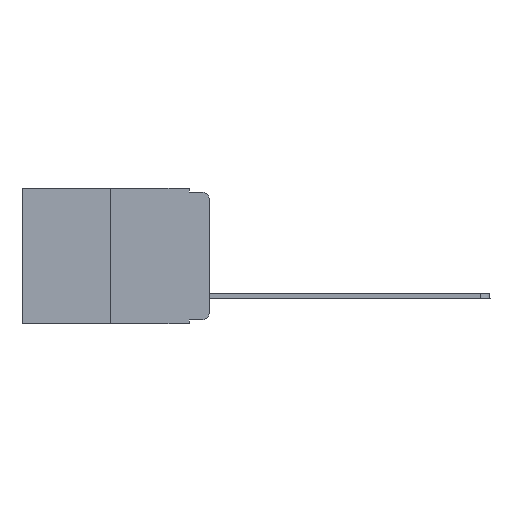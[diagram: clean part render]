
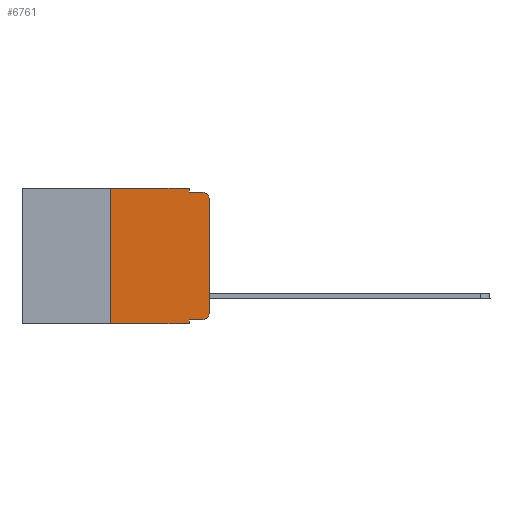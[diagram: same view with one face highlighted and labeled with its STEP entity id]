
A CAD part, left-side view. The second image highlights one B-rep face of the part: STEP entity #6761.
In plain terms, the highlighted planar face has unit normal (-1, 0, 0).
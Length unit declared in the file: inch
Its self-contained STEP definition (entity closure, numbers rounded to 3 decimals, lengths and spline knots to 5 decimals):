
#187 = VECTOR ( 'NONE', #10549, 39.37008 ) ;
#338 = ORIENTED_EDGE ( 'NONE', *, *, #15689, .F. ) ;
#530 = CARTESIAN_POINT ( 'NONE',  ( 0., 0.051, -0.01 ) ) ;
#639 = CARTESIAN_POINT ( 'NONE',  ( 0., 0.02, -0.313 ) ) ;
#808 = LINE ( 'NONE', #20448, #187 ) ;
#814 = CARTESIAN_POINT ( 'NONE',  ( 0., 0.02, -0.01 ) ) ;
#956 = CARTESIAN_POINT ( 'NONE',  ( 0., 0.051, -0.333 ) ) ;
#1038 = LINE ( 'NONE', #530, #24994 ) ;
#1065 = CIRCLE ( 'NONE', #16078, 0.02 ) ;
#1157 = CARTESIAN_POINT ( 'NONE',  ( 0., 0., -0.313 ) ) ;
#1535 = CARTESIAN_POINT ( 'NONE',  ( 0., 0.25, -0.343 ) ) ;
#1928 = VERTEX_POINT ( 'NONE', #956 ) ;
#2062 = EDGE_CURVE ( 'NONE', #1928, #2901, #14173, .T. ) ;
#2238 = ORIENTED_EDGE ( 'NONE', *, *, #15886, .F. ) ;
#2417 = DIRECTION ( 'NONE',  ( 0., 0., -1. ) ) ;
#2697 = DIRECTION ( 'NONE',  ( 0., -1., 0. ) ) ;
#2901 = VERTEX_POINT ( 'NONE', #18277 ) ;
#2909 = FACE_OUTER_BOUND ( 'NONE', #17614, .T. ) ;
#3296 = EDGE_CURVE ( 'NONE', #18042, #2901, #8951, .T. ) ;
#3301 = DIRECTION ( 'NONE',  ( 0., 0., 1. ) ) ;
#3391 = VECTOR ( 'NONE', #15679, 39.37008 ) ;
#4332 = DIRECTION ( 'NONE',  ( 0., 0., -1. ) ) ;
#4492 = DIRECTION ( 'NONE',  ( 0., -1., 0. ) ) ;
#6400 = VERTEX_POINT ( 'NONE', #24580 ) ;
#6761 = ADVANCED_FACE ( 'NONE', ( #2909 ), #8208, .F. ) ;
#6805 = ORIENTED_EDGE ( 'NONE', *, *, #15727, .T. ) ;
#6811 = ORIENTED_EDGE ( 'NONE', *, *, #21255, .F. ) ;
#7413 = VERTEX_POINT ( 'NONE', #14516 ) ;
#8040 = DIRECTION ( 'NONE',  ( 0., -1., 0. ) ) ;
#8192 = LINE ( 'NONE', #18742, #15495 ) ;
#8208 = PLANE ( 'NONE',  #23697 ) ;
#8951 = LINE ( 'NONE', #21450, #3391 ) ;
#9128 = LINE ( 'NONE', #23988, #21363 ) ;
#9532 = CARTESIAN_POINT ( 'NONE',  ( 0., 0.051, 0. ) ) ;
#10383 = CARTESIAN_POINT ( 'NONE',  ( 0., 0.473, 0. ) ) ;
#10549 = DIRECTION ( 'NONE',  ( 0., 0., 1. ) ) ;
#11257 = ORIENTED_EDGE ( 'NONE', *, *, #17722, .T. ) ;
#11288 = DIRECTION ( 'NONE',  ( 0., 0., -1. ) ) ;
#11805 = DIRECTION ( 'NONE',  ( 0., 0., -1. ) ) ;
#11939 = EDGE_CURVE ( 'NONE', #16287, #19735, #808, .T. ) ;
#12506 = CARTESIAN_POINT ( 'NONE',  ( 0., 0., -0.03 ) ) ;
#13027 = DIRECTION ( 'NONE',  ( 0., 0., -1. ) ) ;
#13261 = VERTEX_POINT ( 'NONE', #24370 ) ;
#14048 = DIRECTION ( 'NONE',  ( 1., 0., 0. ) ) ;
#14173 = LINE ( 'NONE', #9532, #18463 ) ;
#14356 = ORIENTED_EDGE ( 'NONE', *, *, #2062, .F. ) ;
#14516 = CARTESIAN_POINT ( 'NONE',  ( 0., 0.051, 0. ) ) ;
#15495 = VECTOR ( 'NONE', #13027, 39.37008 ) ;
#15679 = DIRECTION ( 'NONE',  ( 0., -1., 0. ) ) ;
#15689 = EDGE_CURVE ( 'NONE', #6400, #7413, #25354, .T. ) ;
#15727 = EDGE_CURVE ( 'NONE', #1928, #13261, #9128, .T. ) ;
#15886 = EDGE_CURVE ( 'NONE', #7413, #21447, #8192, .T. ) ;
#16078 = AXIS2_PLACEMENT_3D ( 'NONE', #23483, #21585, #11805 ) ;
#16287 = VERTEX_POINT ( 'NONE', #1157 ) ;
#16294 = DIRECTION ( 'NONE',  ( -1., 0., 0. ) ) ;
#16886 = EDGE_CURVE ( 'NONE', #19735, #23011, #1065, .T. ) ;
#17169 = CARTESIAN_POINT ( 'NONE',  ( 0., 0.25, 0. ) ) ;
#17614 = EDGE_LOOP ( 'NONE', ( #24509, #18765, #6811, #2238, #338, #22087, #23813, #14356, #6805, #11257 ) ) ;
#17722 = EDGE_CURVE ( 'NONE', #13261, #16287, #20961, .T. ) ;
#18042 = VERTEX_POINT ( 'NONE', #1535 ) ;
#18277 = CARTESIAN_POINT ( 'NONE',  ( 0., 0.051, -0.343 ) ) ;
#18463 = VECTOR ( 'NONE', #11288, 39.37008 ) ;
#18742 = CARTESIAN_POINT ( 'NONE',  ( 0., 0.051, 0. ) ) ;
#18765 = ORIENTED_EDGE ( 'NONE', *, *, #16886, .T. ) ;
#18853 = CARTESIAN_POINT ( 'NONE',  ( 0., 0.051, -0.01 ) ) ;
#19735 = VERTEX_POINT ( 'NONE', #12506 ) ;
#20006 = CARTESIAN_POINT ( 'NONE',  ( 0., 0.473, 0. ) ) ;
#20448 = CARTESIAN_POINT ( 'NONE',  ( 0., 0., 0. ) ) ;
#20758 = VECTOR ( 'NONE', #8040, 39.37008 ) ;
#20961 = CIRCLE ( 'NONE', #22689, 0.02 ) ;
#21255 = EDGE_CURVE ( 'NONE', #21447, #23011, #1038, .T. ) ;
#21363 = VECTOR ( 'NONE', #2697, 39.37008 ) ;
#21447 = VERTEX_POINT ( 'NONE', #18853 ) ;
#21450 = CARTESIAN_POINT ( 'NONE',  ( 0., 0.473, -0.343 ) ) ;
#21585 = DIRECTION ( 'NONE',  ( -1., 0., 0. ) ) ;
#22087 = ORIENTED_EDGE ( 'NONE', *, *, #25047, .F. ) ;
#22179 = LINE ( 'NONE', #17169, #23689 ) ;
#22689 = AXIS2_PLACEMENT_3D ( 'NONE', #639, #16294, #4332 ) ;
#23011 = VERTEX_POINT ( 'NONE', #814 ) ;
#23483 = CARTESIAN_POINT ( 'NONE',  ( 0., 0.02, -0.03 ) ) ;
#23689 = VECTOR ( 'NONE', #3301, 39.37008 ) ;
#23697 = AXIS2_PLACEMENT_3D ( 'NONE', #20006, #14048, #2417 ) ;
#23813 = ORIENTED_EDGE ( 'NONE', *, *, #3296, .T. ) ;
#23988 = CARTESIAN_POINT ( 'NONE',  ( 0., 0.051, -0.333 ) ) ;
#24370 = CARTESIAN_POINT ( 'NONE',  ( 0., 0.02, -0.333 ) ) ;
#24509 = ORIENTED_EDGE ( 'NONE', *, *, #11939, .T. ) ;
#24580 = CARTESIAN_POINT ( 'NONE',  ( 0., 0.25, 0. ) ) ;
#24994 = VECTOR ( 'NONE', #4492, 39.37008 ) ;
#25047 = EDGE_CURVE ( 'NONE', #18042, #6400, #22179, .T. ) ;
#25354 = LINE ( 'NONE', #10383, #20758 ) ;
